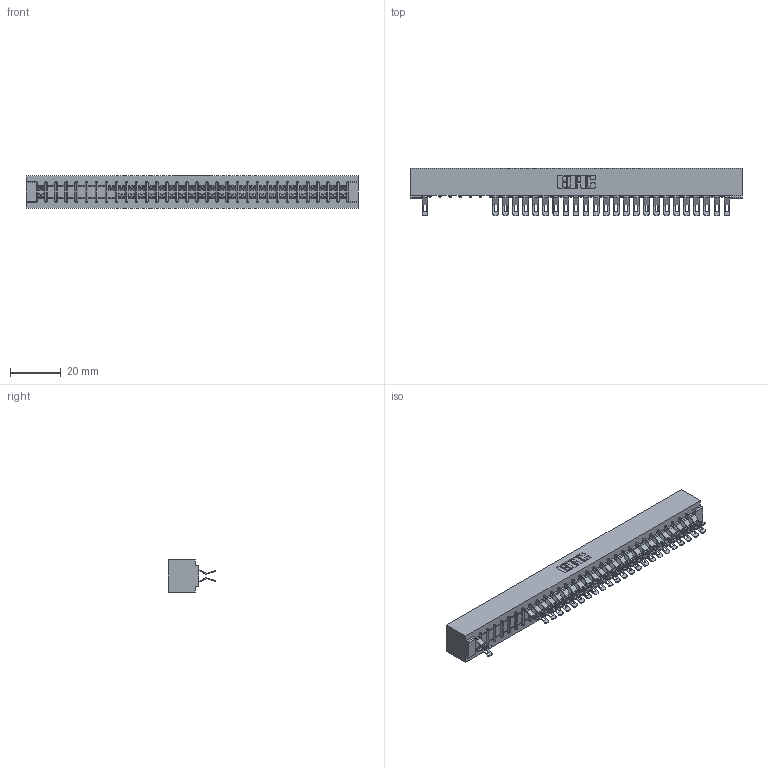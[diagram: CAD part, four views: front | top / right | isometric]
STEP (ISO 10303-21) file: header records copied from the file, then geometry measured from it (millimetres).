
FILE_DESCRIPTION (( 'STEP AP203' ), '1' );
FILE_NAME ('307-062-555-201.STEP', '2018-08-06T09:25:26', ( '' ), ( '' ), 'SwSTEP 2.0', 'SolidWorks 2016', '' );
FILE_SCHEMA (( 'CONFIG_CONTROL_DESIGN' ));
Length unit declared in the file: inch
Products named in the file (3): 307 Part_No Mounting Lugs; 307-290-001_555; 307-062-555-201
Assembly tree (50 placements, depth 2):
  307-062-555-201
    307 Part_No Mounting Lugs
    307-290-001_555  x49
Bounding box: 130.71 x 18.75 x 12.7 mm (x, y, z)
Volume: 14346.6 mm3; surface area: 17351.8 mm2
Topology: 50 solids, 50 shells, 3261 faces, 9584 edges, 6236 vertices
Faces by surface type: plane 1810, cylinder 1387, sphere 64
Entity records: 28767 total; most frequent: CARTESIAN_POINT 4766, ORIENTED_EDGE 4736, DIRECTION 4666, EDGE_CURVE 2368, VECTOR 1802, LINE 1802, VERTEX_POINT 1532, AXIS2_PLACEMENT_3D 1432
